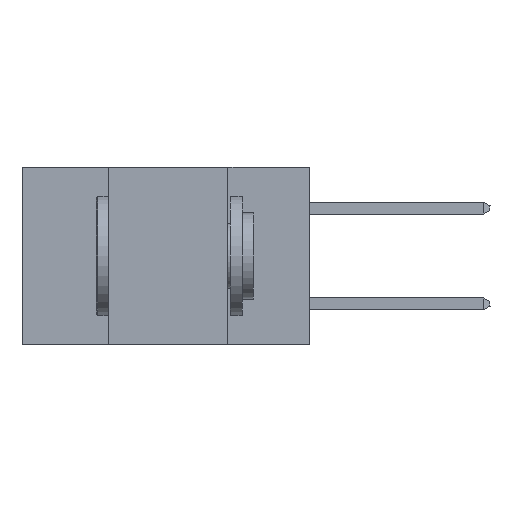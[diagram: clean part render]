
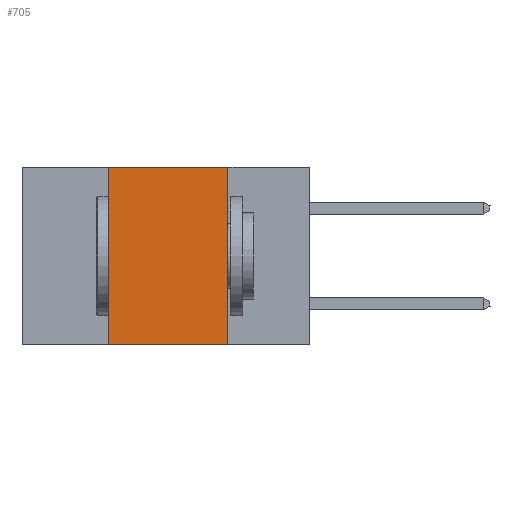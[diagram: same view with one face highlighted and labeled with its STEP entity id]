
A CAD part, left-side view. The second image highlights one B-rep face of the part: STEP entity #705.
In plain terms, the highlighted planar face has unit normal (-1, 0, 0).
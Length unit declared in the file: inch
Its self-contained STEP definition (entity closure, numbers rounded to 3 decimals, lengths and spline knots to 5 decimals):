
#705 = ADVANCED_FACE ( 'NONE', ( #5404 ), #26034, .F. ) ;
#3640 = CARTESIAN_POINT ( 'NONE',  ( 0., 0.17, -0.37 ) ) ;
#5404 = FACE_OUTER_BOUND ( 'NONE', #30050, .T. ) ;
#5895 = ORIENTED_EDGE ( 'NONE', *, *, #18377, .F. ) ;
#6664 = VERTEX_POINT ( 'NONE', #3640 ) ;
#7795 = AXIS2_PLACEMENT_3D ( 'NONE', #14735, #20732, #19849 ) ;
#7926 = LINE ( 'NONE', #16440, #20799 ) ;
#10762 = VERTEX_POINT ( 'NONE', #24884 ) ;
#11991 = CARTESIAN_POINT ( 'NONE',  ( 0., 0.6, -0.37 ) ) ;
#12390 = DIRECTION ( 'NONE',  ( 0., 0., -1. ) ) ;
#12828 = EDGE_CURVE ( 'NONE', #10762, #6664, #17774, .T. ) ;
#13009 = CARTESIAN_POINT ( 'NONE',  ( 0., 0.6, 0. ) ) ;
#13552 = VECTOR ( 'NONE', #23244, 39.37008 ) ;
#14543 = EDGE_CURVE ( 'NONE', #10762, #25083, #7926, .T. ) ;
#14735 = CARTESIAN_POINT ( 'NONE',  ( 0., 0.6, 0. ) ) ;
#16440 = CARTESIAN_POINT ( 'NONE',  ( 0., 0.42, 0. ) ) ;
#17774 = LINE ( 'NONE', #11991, #30355 ) ;
#18377 = EDGE_CURVE ( 'NONE', #23775, #6664, #19331, .T. ) ;
#18956 = DIRECTION ( 'NONE',  ( 0., 0., 1. ) ) ;
#19331 = LINE ( 'NONE', #27598, #20137 ) ;
#19849 = DIRECTION ( 'NONE',  ( 0., 0., -1. ) ) ;
#20137 = VECTOR ( 'NONE', #12390, 39.37008 ) ;
#20308 = LINE ( 'NONE', #13009, #13552 ) ;
#20732 = DIRECTION ( 'NONE',  ( 1., 0., 0. ) ) ;
#20799 = VECTOR ( 'NONE', #18956, 39.37008 ) ;
#23244 = DIRECTION ( 'NONE',  ( 0., -1., 0. ) ) ;
#23596 = ORIENTED_EDGE ( 'NONE', *, *, #14543, .F. ) ;
#23775 = VERTEX_POINT ( 'NONE', #24067 ) ;
#24067 = CARTESIAN_POINT ( 'NONE',  ( 0., 0.17, 0. ) ) ;
#24884 = CARTESIAN_POINT ( 'NONE',  ( 0., 0.42, -0.37 ) ) ;
#25083 = VERTEX_POINT ( 'NONE', #27436 ) ;
#25202 = ORIENTED_EDGE ( 'NONE', *, *, #12828, .T. ) ;
#26034 = PLANE ( 'NONE',  #7795 ) ;
#27068 = EDGE_CURVE ( 'NONE', #25083, #23775, #20308, .T. ) ;
#27221 = DIRECTION ( 'NONE',  ( 0., -1., 0. ) ) ;
#27436 = CARTESIAN_POINT ( 'NONE',  ( 0., 0.42, 0. ) ) ;
#27598 = CARTESIAN_POINT ( 'NONE',  ( 0., 0.17, 0. ) ) ;
#29473 = ORIENTED_EDGE ( 'NONE', *, *, #27068, .F. ) ;
#30050 = EDGE_LOOP ( 'NONE', ( #5895, #29473, #23596, #25202 ) ) ;
#30355 = VECTOR ( 'NONE', #27221, 39.37008 ) ;
